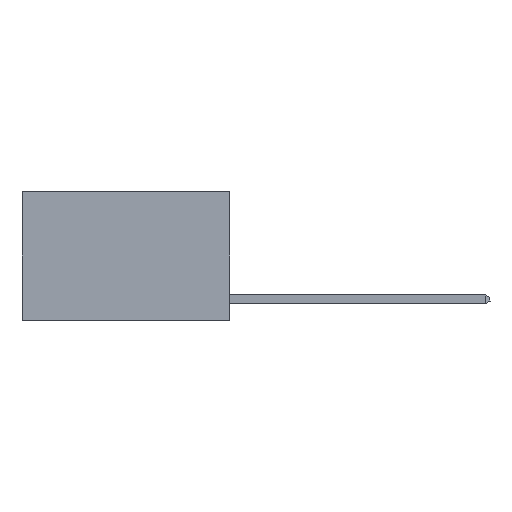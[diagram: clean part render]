
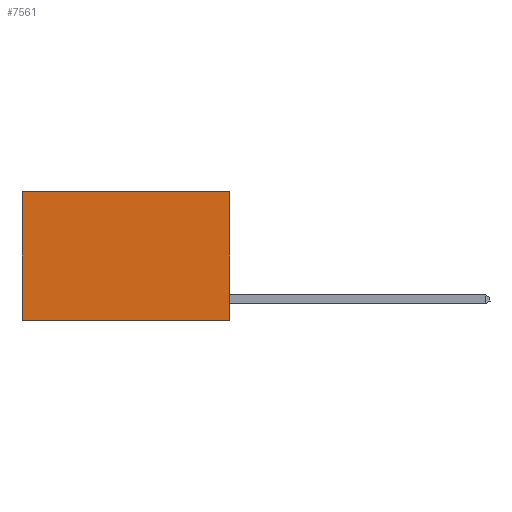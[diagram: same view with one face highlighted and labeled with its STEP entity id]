
A CAD part, left-side view. The second image highlights one B-rep face of the part: STEP entity #7561.
In plain terms, the highlighted planar face has unit normal (-1, 0, 0).
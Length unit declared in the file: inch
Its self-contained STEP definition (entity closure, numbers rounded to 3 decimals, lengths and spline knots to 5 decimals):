
#258 = DIRECTION ( 'NONE',  ( 0., 1., 0. ) ) ;
#369 = FACE_OUTER_BOUND ( 'NONE', #15621, .T. ) ;
#375 = CARTESIAN_POINT ( 'NONE',  ( 0.2625, 0., -0.37 ) ) ;
#769 = VECTOR ( 'NONE', #1315, 39.37008 ) ;
#857 = VERTEX_POINT ( 'NONE', #15123 ) ;
#886 = EDGE_CURVE ( 'NONE', #857, #12612, #14984, .T. ) ;
#1131 = ORIENTED_EDGE ( 'NONE', *, *, #6207, .F. ) ;
#1315 = DIRECTION ( 'NONE',  ( 0., 1., 0. ) ) ;
#1512 = LINE ( 'NONE', #8470, #13096 ) ;
#1619 = EDGE_CURVE ( 'NONE', #3409, #2053, #4401, .T. ) ;
#1691 = CARTESIAN_POINT ( 'NONE',  ( 0.2625, 0., 0. ) ) ;
#2053 = VERTEX_POINT ( 'NONE', #2687 ) ;
#2638 = CARTESIAN_POINT ( 'NONE',  ( 0.2625, 0.6, 0. ) ) ;
#2687 = CARTESIAN_POINT ( 'NONE',  ( 0.2625, 0.6, -0.37 ) ) ;
#3409 = VERTEX_POINT ( 'NONE', #11854 ) ;
#4401 = LINE ( 'NONE', #375, #6019 ) ;
#5558 = AXIS2_PLACEMENT_3D ( 'NONE', #6087, #13908, #11320 ) ;
#6019 = VECTOR ( 'NONE', #258, 39.37008 ) ;
#6087 = CARTESIAN_POINT ( 'NONE',  ( 0.2625, 0., 0. ) ) ;
#6207 = EDGE_CURVE ( 'NONE', #857, #3409, #14613, .T. ) ;
#6394 = CARTESIAN_POINT ( 'NONE',  ( 0.2625, 0., 0. ) ) ;
#6474 = ORIENTED_EDGE ( 'NONE', *, *, #1619, .F. ) ;
#6724 = DIRECTION ( 'NONE',  ( 0., 0., -1. ) ) ;
#7561 = ADVANCED_FACE ( 'NONE', ( #369 ), #9842, .F. ) ;
#8470 = CARTESIAN_POINT ( 'NONE',  ( 0.2625, 0.6, 0. ) ) ;
#9288 = EDGE_CURVE ( 'NONE', #12612, #2053, #1512, .T. ) ;
#9842 = PLANE ( 'NONE',  #5558 ) ;
#11320 = DIRECTION ( 'NONE',  ( 0., 0., -1. ) ) ;
#11854 = CARTESIAN_POINT ( 'NONE',  ( 0.2625, 0., -0.37 ) ) ;
#12155 = ORIENTED_EDGE ( 'NONE', *, *, #9288, .T. ) ;
#12160 = DIRECTION ( 'NONE',  ( 0., 0., -1. ) ) ;
#12612 = VERTEX_POINT ( 'NONE', #2638 ) ;
#12816 = VECTOR ( 'NONE', #6724, 39.37008 ) ;
#12991 = ORIENTED_EDGE ( 'NONE', *, *, #886, .T. ) ;
#13096 = VECTOR ( 'NONE', #12160, 39.37008 ) ;
#13908 = DIRECTION ( 'NONE',  ( 1., 0., 0. ) ) ;
#14613 = LINE ( 'NONE', #1691, #12816 ) ;
#14984 = LINE ( 'NONE', #6394, #769 ) ;
#15123 = CARTESIAN_POINT ( 'NONE',  ( 0.2625, 0., 0. ) ) ;
#15621 = EDGE_LOOP ( 'NONE', ( #12155, #6474, #1131, #12991 ) ) ;
